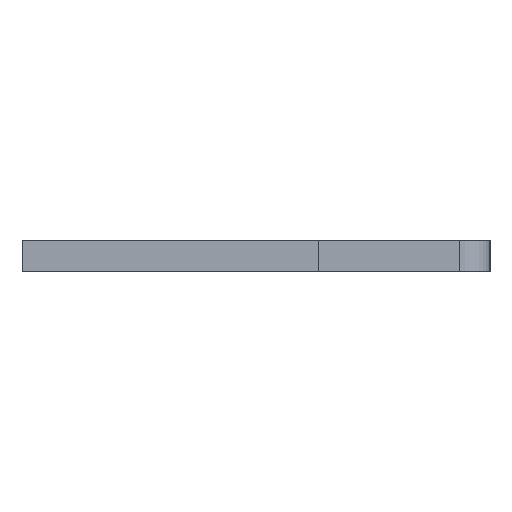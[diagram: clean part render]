
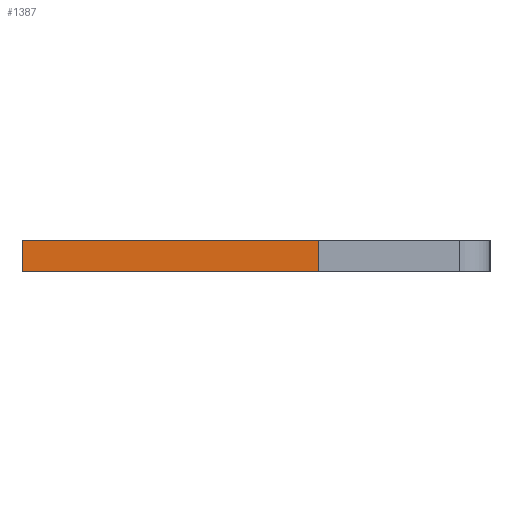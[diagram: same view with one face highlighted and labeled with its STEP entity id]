
A CAD part, left-side view. The second image highlights one B-rep face of the part: STEP entity #1387.
In plain terms, the highlighted face is planar.
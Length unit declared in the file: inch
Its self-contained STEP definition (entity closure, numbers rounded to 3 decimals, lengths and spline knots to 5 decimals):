
#19 = CARTESIAN_POINT ( 'NONE',  ( -0.01, -0.04, -0.04 ) ) ;
#21 = AXIS2_PLACEMENT_3D ( 'NONE', #809, #139, #27 ) ;
#27 = DIRECTION ( 'NONE',  ( 1., 0., 0. ) ) ;
#44 = LINE ( 'NONE', #1115, #391 ) ;
#93 = VECTOR ( 'NONE', #1129, 39.37008 ) ;
#105 = CARTESIAN_POINT ( 'NONE',  ( 0.01, 0.15, -0.04 ) ) ;
#117 = ORIENTED_EDGE ( 'NONE', *, *, #1222, .T. ) ;
#139 = DIRECTION ( 'NONE',  ( 0., 0., 1. ) ) ;
#158 = EDGE_LOOP ( 'NONE', ( #117, #1196, #929, #1194 ) ) ;
#162 = VECTOR ( 'NONE', #1118, 39.37008 ) ;
#177 = DIRECTION ( 'NONE',  ( -1., 0., 0. ) ) ;
#212 = CARTESIAN_POINT ( 'NONE',  ( 0.01, -0.04, -0.04 ) ) ;
#374 = FACE_OUTER_BOUND ( 'NONE', #158, .T. ) ;
#391 = VECTOR ( 'NONE', #785, 39.37008 ) ;
#566 = CARTESIAN_POINT ( 'NONE',  ( 0.01, 0.15, -0.04 ) ) ;
#593 = LINE ( 'NONE', #846, #907 ) ;
#665 = EDGE_CURVE ( 'NONE', #1083, #1354, #593, .T. ) ;
#742 = LINE ( 'NONE', #566, #93 ) ;
#785 = DIRECTION ( 'NONE',  ( 0., 1., 0. ) ) ;
#791 = CARTESIAN_POINT ( 'NONE',  ( 0.01, 0.15, -0.04 ) ) ;
#809 = CARTESIAN_POINT ( 'NONE',  ( 0.01, 0.15, -0.04 ) ) ;
#846 = CARTESIAN_POINT ( 'NONE',  ( 0.01, -0.04, -0.04 ) ) ;
#905 = PLANE ( 'NONE',  #21 ) ;
#907 = VECTOR ( 'NONE', #177, 39.37008 ) ;
#929 = ORIENTED_EDGE ( 'NONE', *, *, #941, .F. ) ;
#941 = EDGE_CURVE ( 'NONE', #1083, #1037, #978, .T. ) ;
#978 = LINE ( 'NONE', #791, #162 ) ;
#1037 = VERTEX_POINT ( 'NONE', #105 ) ;
#1083 = VERTEX_POINT ( 'NONE', #212 ) ;
#1115 = CARTESIAN_POINT ( 'NONE',  ( -0.01, 0.15, -0.04 ) ) ;
#1118 = DIRECTION ( 'NONE',  ( 0., 1., 0. ) ) ;
#1122 = EDGE_CURVE ( 'NONE', #1037, #1128, #742, .T. ) ;
#1128 = VERTEX_POINT ( 'NONE', #1362 ) ;
#1129 = DIRECTION ( 'NONE',  ( -1., 0., 0. ) ) ;
#1194 = ORIENTED_EDGE ( 'NONE', *, *, #665, .T. ) ;
#1196 = ORIENTED_EDGE ( 'NONE', *, *, #1122, .F. ) ;
#1222 = EDGE_CURVE ( 'NONE', #1354, #1128, #44, .T. ) ;
#1354 = VERTEX_POINT ( 'NONE', #19 ) ;
#1362 = CARTESIAN_POINT ( 'NONE',  ( -0.01, 0.15, -0.04 ) ) ;
#1387 = ADVANCED_FACE ( 'NONE', ( #374 ), #905, .F. ) ;
